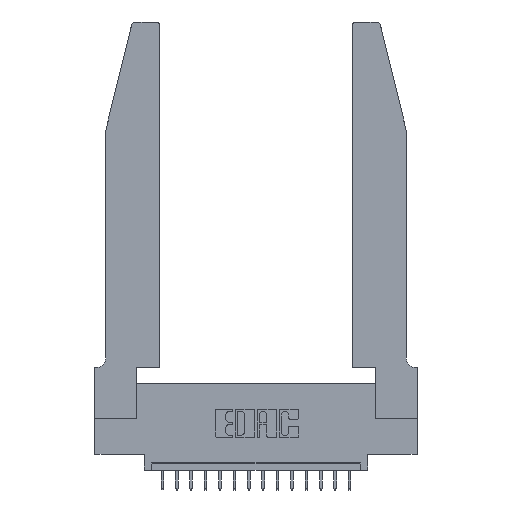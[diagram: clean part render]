
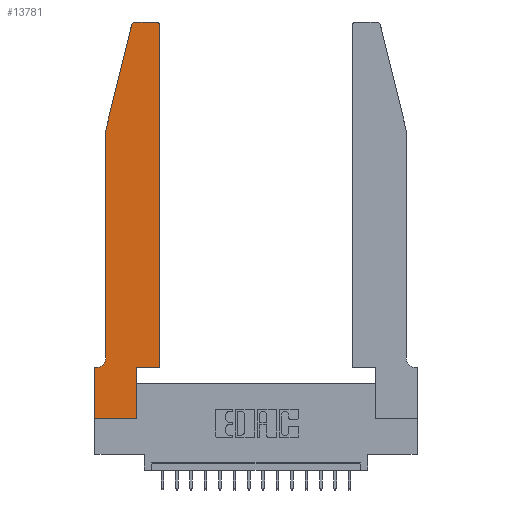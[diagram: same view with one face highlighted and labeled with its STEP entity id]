
A CAD part, top view. The second image highlights one B-rep face of the part: STEP entity #13781.
In plain terms, the highlighted planar face has unit normal (0, 0, 1).
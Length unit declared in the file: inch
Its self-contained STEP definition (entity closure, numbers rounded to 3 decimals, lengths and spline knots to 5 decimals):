
#3 = VERTEX_POINT ( 'NONE', #13030 ) ;
#275 = DIRECTION ( 'NONE',  ( 1., 0., 0. ) ) ;
#692 = EDGE_CURVE ( 'NONE', #15011, #14117, #8553, .T. ) ;
#741 = DIRECTION ( 'NONE',  ( -1., 0., 0. ) ) ;
#797 = CARTESIAN_POINT ( 'NONE',  ( 0.0055, 0.42, 0.37 ) ) ;
#1293 = DIRECTION ( 'NONE',  ( 0., -1., 0. ) ) ;
#1587 = ORIENTED_EDGE ( 'NONE', *, *, #2976, .T. ) ;
#2596 = VERTEX_POINT ( 'NONE', #5997 ) ;
#2976 = EDGE_CURVE ( 'NONE', #2596, #3, #18745, .T. ) ;
#3389 = EDGE_CURVE ( 'NONE', #11994, #9730, #10292, .T. ) ;
#3686 = CARTESIAN_POINT ( 'NONE',  ( 0.0755, 0.42, 0.37 ) ) ;
#3695 = DIRECTION ( 'NONE',  ( 1., 0., 0. ) ) ;
#4338 = DIRECTION ( 'NONE',  ( 0., 1., 0. ) ) ;
#4446 = VECTOR ( 'NONE', #12360, 39.37008 ) ;
#4520 = VERTEX_POINT ( 'NONE', #12663 ) ;
#4587 = CARTESIAN_POINT ( 'NONE',  ( 0., 0., 0.37 ) ) ;
#4670 = VERTEX_POINT ( 'NONE', #9425 ) ;
#4734 = VECTOR ( 'NONE', #4338, 39.37008 ) ;
#4793 = ORIENTED_EDGE ( 'NONE', *, *, #16999, .T. ) ;
#4832 = LINE ( 'NONE', #15369, #6417 ) ;
#5254 = LINE ( 'NONE', #18841, #4734 ) ;
#5349 = ORIENTED_EDGE ( 'NONE', *, *, #7090, .T. ) ;
#5997 = CARTESIAN_POINT ( 'NONE',  ( 0.2865, 0.35, 0.37 ) ) ;
#5999 = VERTEX_POINT ( 'NONE', #13385 ) ;
#6417 = VECTOR ( 'NONE', #741, 39.37008 ) ;
#6610 = AXIS2_PLACEMENT_3D ( 'NONE', #17157, #6897, #3695 ) ;
#6897 = DIRECTION ( 'NONE',  ( 0., 0., 1. ) ) ;
#7090 = EDGE_CURVE ( 'NONE', #4670, #15963, #10957, .T. ) ;
#7129 = CARTESIAN_POINT ( 'NONE',  ( 0., 0., 0.37 ) ) ;
#7183 = EDGE_CURVE ( 'NONE', #14287, #5999, #8125, .T. ) ;
#7213 = VECTOR ( 'NONE', #16170, 39.37008 ) ;
#7259 = AXIS2_PLACEMENT_3D ( 'NONE', #13164, #19115, #8674 ) ;
#7490 = ORIENTED_EDGE ( 'NONE', *, *, #12748, .T. ) ;
#7874 = CARTESIAN_POINT ( 'NONE',  ( 0.4505, 0.35, 0.37 ) ) ;
#8125 = CIRCLE ( 'NONE', #10282, 0.03 ) ;
#8439 = CARTESIAN_POINT ( 'NONE',  ( 0.0755, 0.35, 0.37 ) ) ;
#8486 = DIRECTION ( 'NONE',  ( 1., 0., 0. ) ) ;
#8532 = EDGE_CURVE ( 'NONE', #5999, #4670, #16263, .T. ) ;
#8553 = LINE ( 'NONE', #8439, #18536 ) ;
#8674 = DIRECTION ( 'NONE',  ( 1., 0., 0. ) ) ;
#8696 = VECTOR ( 'NONE', #8486, 39.37008 ) ;
#8771 = ORIENTED_EDGE ( 'NONE', *, *, #7183, .T. ) ;
#9016 = CARTESIAN_POINT ( 'NONE',  ( 0.284, 2.72, 0.37 ) ) ;
#9201 = ORIENTED_EDGE ( 'NONE', *, *, #8532, .T. ) ;
#9279 = DIRECTION ( 'NONE',  ( 0., 0., -1. ) ) ;
#9352 = EDGE_LOOP ( 'NONE', ( #17337, #8771, #9201, #5349, #4793, #13876, #16500, #11121, #16515, #1587, #13245, #7490 ) ) ;
#9358 = LINE ( 'NONE', #7874, #4446 ) ;
#9425 = CARTESIAN_POINT ( 'NONE',  ( 0.0755, 2., 0.37 ) ) ;
#9631 = VECTOR ( 'NONE', #275, 39.37008 ) ;
#9730 = VERTEX_POINT ( 'NONE', #15811 ) ;
#9960 = EDGE_CURVE ( 'NONE', #3, #13072, #9358, .T. ) ;
#10008 = DIRECTION ( 'NONE',  ( -1., 0., 0. ) ) ;
#10191 = CARTESIAN_POINT ( 'NONE',  ( 0.0755, 2., 0.37 ) ) ;
#10282 = AXIS2_PLACEMENT_3D ( 'NONE', #9016, #16345, #13409 ) ;
#10292 = LINE ( 'NONE', #13637, #9631 ) ;
#10912 = VECTOR ( 'NONE', #14007, 39.37008 ) ;
#10957 = LINE ( 'NONE', #15477, #10912 ) ;
#11121 = ORIENTED_EDGE ( 'NONE', *, *, #3389, .T. ) ;
#11138 = EDGE_CURVE ( 'NONE', #9730, #2596, #5254, .T. ) ;
#11682 = CARTESIAN_POINT ( 'NONE',  ( 0.4505, 0.35, 0.37 ) ) ;
#11994 = VERTEX_POINT ( 'NONE', #4587 ) ;
#12360 = DIRECTION ( 'NONE',  ( 0., 1., 0. ) ) ;
#12581 = EDGE_CURVE ( 'NONE', #14117, #11994, #13297, .T. ) ;
#12663 = CARTESIAN_POINT ( 'NONE',  ( 0.4205, 2.75, 0.37 ) ) ;
#12748 = EDGE_CURVE ( 'NONE', #13072, #4520, #14450, .T. ) ;
#12901 = VECTOR ( 'NONE', #1293, 39.37008 ) ;
#13030 = CARTESIAN_POINT ( 'NONE',  ( 0.4505, 0.35, 0.37 ) ) ;
#13072 = VERTEX_POINT ( 'NONE', #18074 ) ;
#13164 = CARTESIAN_POINT ( 'NONE',  ( 0.4205, 2.72, 0.37 ) ) ;
#13245 = ORIENTED_EDGE ( 'NONE', *, *, #9960, .T. ) ;
#13297 = LINE ( 'NONE', #7129, #12901 ) ;
#13385 = CARTESIAN_POINT ( 'NONE',  ( 0.25487, 2.72718, 0.37 ) ) ;
#13409 = DIRECTION ( 'NONE',  ( 1., 0., 0. ) ) ;
#13615 = CIRCLE ( 'NONE', #17022, 0.07 ) ;
#13637 = CARTESIAN_POINT ( 'NONE',  ( 0., 0., 0.37 ) ) ;
#13781 = ADVANCED_FACE ( 'NONE', ( #17266 ), #14152, .T. ) ;
#13876 = ORIENTED_EDGE ( 'NONE', *, *, #692, .T. ) ;
#14007 = DIRECTION ( 'NONE',  ( 0., -1., 0. ) ) ;
#14117 = VERTEX_POINT ( 'NONE', #14573 ) ;
#14152 = PLANE ( 'NONE',  #6610 ) ;
#14287 = VERTEX_POINT ( 'NONE', #16513 ) ;
#14450 = CIRCLE ( 'NONE', #7259, 0.03 ) ;
#14573 = CARTESIAN_POINT ( 'NONE',  ( 0., 0.35, 0.37 ) ) ;
#14993 = CARTESIAN_POINT ( 'NONE',  ( 0.0055, 0.35, 0.37 ) ) ;
#15011 = VERTEX_POINT ( 'NONE', #14993 ) ;
#15226 = DIRECTION ( 'NONE',  ( -1., 0., 0. ) ) ;
#15369 = CARTESIAN_POINT ( 'NONE',  ( 0.2605, 2.75, 0.37 ) ) ;
#15477 = CARTESIAN_POINT ( 'NONE',  ( 0.0755, 2., 0.37 ) ) ;
#15811 = CARTESIAN_POINT ( 'NONE',  ( 0.2865, 0., 0.37 ) ) ;
#15963 = VERTEX_POINT ( 'NONE', #3686 ) ;
#16170 = DIRECTION ( 'NONE',  ( -0.239, -0.971, 0. ) ) ;
#16263 = LINE ( 'NONE', #10191, #7213 ) ;
#16345 = DIRECTION ( 'NONE',  ( 0., 0., 1. ) ) ;
#16375 = EDGE_CURVE ( 'NONE', #4520, #14287, #4832, .T. ) ;
#16500 = ORIENTED_EDGE ( 'NONE', *, *, #12581, .T. ) ;
#16513 = CARTESIAN_POINT ( 'NONE',  ( 0.284, 2.75, 0.37 ) ) ;
#16515 = ORIENTED_EDGE ( 'NONE', *, *, #11138, .T. ) ;
#16999 = EDGE_CURVE ( 'NONE', #15963, #15011, #13615, .T. ) ;
#17022 = AXIS2_PLACEMENT_3D ( 'NONE', #797, #9279, #15226 ) ;
#17157 = CARTESIAN_POINT ( 'NONE',  ( 0., 0.35, 0.37 ) ) ;
#17266 = FACE_OUTER_BOUND ( 'NONE', #9352, .T. ) ;
#17337 = ORIENTED_EDGE ( 'NONE', *, *, #16375, .T. ) ;
#18074 = CARTESIAN_POINT ( 'NONE',  ( 0.4505, 2.72, 0.37 ) ) ;
#18536 = VECTOR ( 'NONE', #10008, 39.37008 ) ;
#18745 = LINE ( 'NONE', #11682, #8696 ) ;
#18841 = CARTESIAN_POINT ( 'NONE',  ( 0.2865, 0.35, 0.37 ) ) ;
#19115 = DIRECTION ( 'NONE',  ( 0., 0., 1. ) ) ;
